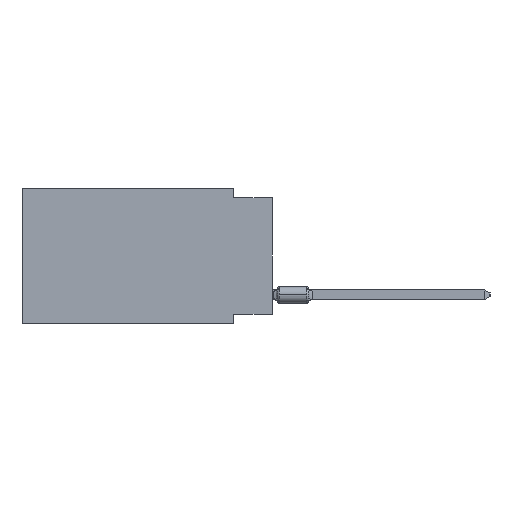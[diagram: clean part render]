
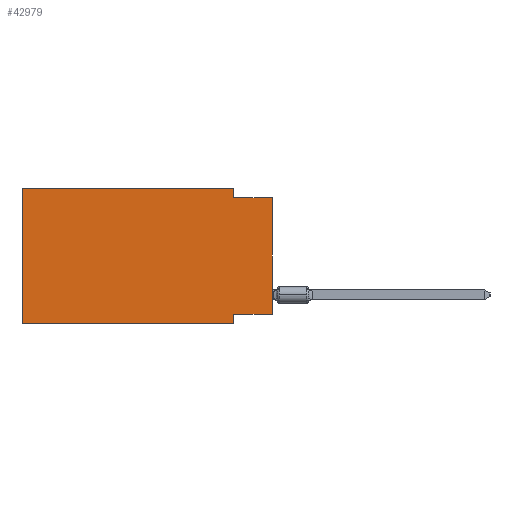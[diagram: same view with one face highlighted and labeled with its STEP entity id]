
A CAD part, left-side view. The second image highlights one B-rep face of the part: STEP entity #42979.
In plain terms, the highlighted planar face has unit normal (-1, 0, 0).
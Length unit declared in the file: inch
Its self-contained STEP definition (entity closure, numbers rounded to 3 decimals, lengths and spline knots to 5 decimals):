
#455 = EDGE_CURVE ( 'NONE', #47912, #36332, #36019, .T. ) ;
#1169 = CARTESIAN_POINT ( 'NONE',  ( 0., 0.645, 0. ) ) ;
#2228 = VECTOR ( 'NONE', #5763, 39.37008 ) ;
#2312 = CARTESIAN_POINT ( 'NONE',  ( 0., 0.645, -0.35 ) ) ;
#3687 = DIRECTION ( 'NONE',  ( 0., 0., 1. ) ) ;
#5763 = DIRECTION ( 'NONE',  ( 0., 0., -1. ) ) ;
#6233 = VECTOR ( 'NONE', #49466, 39.37008 ) ;
#6293 = VECTOR ( 'NONE', #3687, 39.37008 ) ;
#6647 = AXIS2_PLACEMENT_3D ( 'NONE', #65359, #39611, #18897 ) ;
#6719 = CARTESIAN_POINT ( 'NONE',  ( 0., 0.1, -0.325 ) ) ;
#7319 = CARTESIAN_POINT ( 'NONE',  ( 0., 0.1, -0.025 ) ) ;
#8079 = EDGE_CURVE ( 'NONE', #59604, #34771, #25408, .T. ) ;
#8700 = CARTESIAN_POINT ( 'NONE',  ( 0., 0.645, 0. ) ) ;
#8725 = LINE ( 'NONE', #64859, #6233 ) ;
#9637 = EDGE_CURVE ( 'NONE', #50897, #59170, #27374, .T. ) ;
#10192 = VECTOR ( 'NONE', #55735, 39.37008 ) ;
#11284 = CARTESIAN_POINT ( 'NONE',  ( 0., 0., -0.325 ) ) ;
#15139 = CARTESIAN_POINT ( 'NONE',  ( 0., 0.1, 0. ) ) ;
#15919 = CARTESIAN_POINT ( 'NONE',  ( 0., 0.645, 0. ) ) ;
#16920 = CARTESIAN_POINT ( 'NONE',  ( 0., 0., -0.025 ) ) ;
#17404 = EDGE_CURVE ( 'NONE', #34771, #53981, #61683, .T. ) ;
#18897 = DIRECTION ( 'NONE',  ( 0., 0., -1. ) ) ;
#19011 = ORIENTED_EDGE ( 'NONE', *, *, #9637, .T. ) ;
#19166 = CARTESIAN_POINT ( 'NONE',  ( 0., 0.1, -0.35 ) ) ;
#22380 = DIRECTION ( 'NONE',  ( 0., 0., 1. ) ) ;
#22846 = VERTEX_POINT ( 'NONE', #7319 ) ;
#23544 = ORIENTED_EDGE ( 'NONE', *, *, #36709, .F. ) ;
#25408 = LINE ( 'NONE', #8700, #6293 ) ;
#27374 = LINE ( 'NONE', #48388, #35635 ) ;
#27385 = LINE ( 'NONE', #2312, #46632 ) ;
#28524 = EDGE_LOOP ( 'NONE', ( #19011, #41112, #40741, #32584, #65593, #29698, #57556, #23544 ) ) ;
#29698 = ORIENTED_EDGE ( 'NONE', *, *, #64786, .T. ) ;
#30310 = CARTESIAN_POINT ( 'NONE',  ( 0., 0., -0.025 ) ) ;
#31263 = DIRECTION ( 'NONE',  ( 0., -1., 0. ) ) ;
#31434 = CARTESIAN_POINT ( 'NONE',  ( 0., 0.1, 0. ) ) ;
#32584 = ORIENTED_EDGE ( 'NONE', *, *, #17404, .F. ) ;
#32586 = DIRECTION ( 'NONE',  ( 0., -1., 0. ) ) ;
#34269 = FACE_OUTER_BOUND ( 'NONE', #28524, .T. ) ;
#34771 = VERTEX_POINT ( 'NONE', #1169 ) ;
#35635 = VECTOR ( 'NONE', #22380, 39.37008 ) ;
#36019 = LINE ( 'NONE', #51377, #10192 ) ;
#36332 = VERTEX_POINT ( 'NONE', #19166 ) ;
#36709 = EDGE_CURVE ( 'NONE', #50897, #47912, #8725, .T. ) ;
#39611 = DIRECTION ( 'NONE',  ( 1., 0., 0. ) ) ;
#40741 = ORIENTED_EDGE ( 'NONE', *, *, #41837, .F. ) ;
#40792 = EDGE_CURVE ( 'NONE', #22846, #59170, #57676, .T. ) ;
#41112 = ORIENTED_EDGE ( 'NONE', *, *, #40792, .F. ) ;
#41494 = CARTESIAN_POINT ( 'NONE',  ( 0., 0.645, -0.35 ) ) ;
#41837 = EDGE_CURVE ( 'NONE', #53981, #22846, #49603, .T. ) ;
#42979 = ADVANCED_FACE ( 'NONE', ( #34269 ), #44962, .F. ) ;
#44962 = PLANE ( 'NONE',  #6647 ) ;
#46632 = VECTOR ( 'NONE', #63143, 39.37008 ) ;
#47912 = VERTEX_POINT ( 'NONE', #6719 ) ;
#48388 = CARTESIAN_POINT ( 'NONE',  ( 0., 0., 0. ) ) ;
#49466 = DIRECTION ( 'NONE',  ( 0., 1., 0. ) ) ;
#49603 = LINE ( 'NONE', #15139, #2228 ) ;
#50897 = VERTEX_POINT ( 'NONE', #11284 ) ;
#51377 = CARTESIAN_POINT ( 'NONE',  ( 0., 0.1, -0.35 ) ) ;
#53981 = VERTEX_POINT ( 'NONE', #31434 ) ;
#55735 = DIRECTION ( 'NONE',  ( 0., 0., -1. ) ) ;
#57556 = ORIENTED_EDGE ( 'NONE', *, *, #455, .F. ) ;
#57676 = LINE ( 'NONE', #16920, #59752 ) ;
#59170 = VERTEX_POINT ( 'NONE', #30310 ) ;
#59604 = VERTEX_POINT ( 'NONE', #41494 ) ;
#59752 = VECTOR ( 'NONE', #32586, 39.37008 ) ;
#61683 = LINE ( 'NONE', #15919, #62958 ) ;
#62958 = VECTOR ( 'NONE', #31263, 39.37008 ) ;
#63143 = DIRECTION ( 'NONE',  ( 0., -1., 0. ) ) ;
#64786 = EDGE_CURVE ( 'NONE', #59604, #36332, #27385, .T. ) ;
#64859 = CARTESIAN_POINT ( 'NONE',  ( 0., 0., -0.325 ) ) ;
#65359 = CARTESIAN_POINT ( 'NONE',  ( 0., 0.645, 0. ) ) ;
#65593 = ORIENTED_EDGE ( 'NONE', *, *, #8079, .F. ) ;
